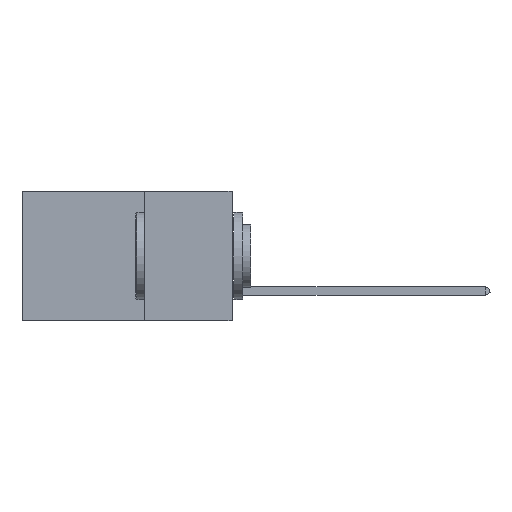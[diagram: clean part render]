
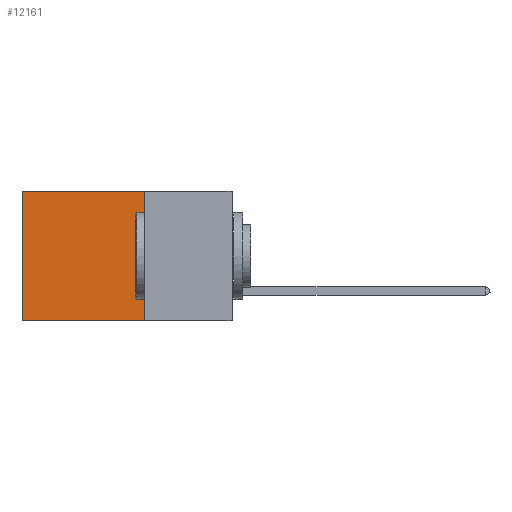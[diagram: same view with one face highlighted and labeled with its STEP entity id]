
A CAD part, left-side view. The second image highlights one B-rep face of the part: STEP entity #12161.
In plain terms, the highlighted planar face has unit normal (-1, 0, 0).
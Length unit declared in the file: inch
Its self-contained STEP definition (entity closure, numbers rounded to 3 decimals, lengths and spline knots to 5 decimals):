
#325 = CARTESIAN_POINT ( 'NONE',  ( 0.2875, 0.6, 0. ) ) ;
#3088 = FACE_OUTER_BOUND ( 'NONE', #21440, .T. ) ;
#3720 = LINE ( 'NONE', #28962, #21365 ) ;
#3783 = CARTESIAN_POINT ( 'NONE',  ( 0.2875, 0.6, -0.37 ) ) ;
#4369 = VERTEX_POINT ( 'NONE', #26194 ) ;
#4406 = EDGE_CURVE ( 'NONE', #4369, #8650, #17246, .T. ) ;
#5363 = AXIS2_PLACEMENT_3D ( 'NONE', #5903, #22153, #29137 ) ;
#5541 = DIRECTION ( 'NONE',  ( 0., 1., 0. ) ) ;
#5903 = CARTESIAN_POINT ( 'NONE',  ( 0.2875, 0.25, 0. ) ) ;
#6618 = CARTESIAN_POINT ( 'NONE',  ( 0.2875, 0.25, -0.37 ) ) ;
#7100 = VECTOR ( 'NONE', #17469, 39.37008 ) ;
#7249 = LINE ( 'NONE', #12840, #10566 ) ;
#7714 = CARTESIAN_POINT ( 'NONE',  ( 0.2875, 0.25, 0. ) ) ;
#7769 = ORIENTED_EDGE ( 'NONE', *, *, #21779, .T. ) ;
#8650 = VERTEX_POINT ( 'NONE', #3783 ) ;
#10566 = VECTOR ( 'NONE', #12945, 39.37008 ) ;
#10677 = EDGE_CURVE ( 'NONE', #29788, #28673, #25858, .T. ) ;
#12161 = ADVANCED_FACE ( 'NONE', ( #3088 ), #17186, .F. ) ;
#12840 = CARTESIAN_POINT ( 'NONE',  ( 0.2875, 0.25, -0.37 ) ) ;
#12945 = DIRECTION ( 'NONE',  ( 0., 1., 0. ) ) ;
#16268 = EDGE_CURVE ( 'NONE', #28673, #8650, #7249, .T. ) ;
#17186 = PLANE ( 'NONE',  #5363 ) ;
#17246 = LINE ( 'NONE', #325, #24276 ) ;
#17469 = DIRECTION ( 'NONE',  ( 0., 0., -1. ) ) ;
#17682 = ORIENTED_EDGE ( 'NONE', *, *, #10677, .F. ) ;
#18497 = ORIENTED_EDGE ( 'NONE', *, *, #4406, .T. ) ;
#21365 = VECTOR ( 'NONE', #5541, 39.37008 ) ;
#21440 = EDGE_LOOP ( 'NONE', ( #18497, #29898, #17682, #7769 ) ) ;
#21779 = EDGE_CURVE ( 'NONE', #29788, #4369, #3720, .T. ) ;
#22153 = DIRECTION ( 'NONE',  ( 1., 0., 0. ) ) ;
#24276 = VECTOR ( 'NONE', #26513, 39.37008 ) ;
#25858 = LINE ( 'NONE', #7714, #7100 ) ;
#26194 = CARTESIAN_POINT ( 'NONE',  ( 0.2875, 0.6, 0. ) ) ;
#26513 = DIRECTION ( 'NONE',  ( 0., 0., -1. ) ) ;
#28673 = VERTEX_POINT ( 'NONE', #6618 ) ;
#28962 = CARTESIAN_POINT ( 'NONE',  ( 0.2875, 0.25, 0. ) ) ;
#29137 = DIRECTION ( 'NONE',  ( 0., 0., -1. ) ) ;
#29376 = CARTESIAN_POINT ( 'NONE',  ( 0.2875, 0.25, 0. ) ) ;
#29788 = VERTEX_POINT ( 'NONE', #29376 ) ;
#29898 = ORIENTED_EDGE ( 'NONE', *, *, #16268, .F. ) ;
